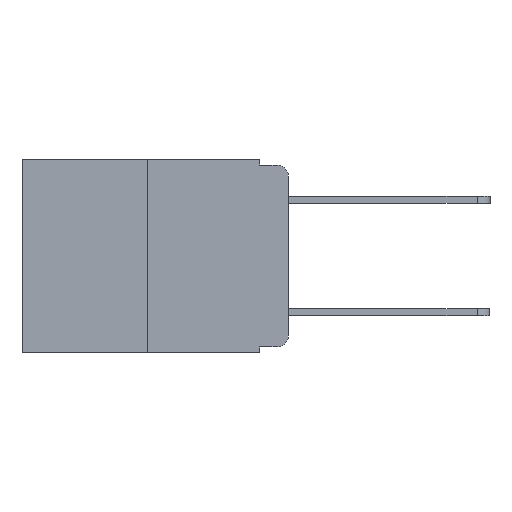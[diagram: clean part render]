
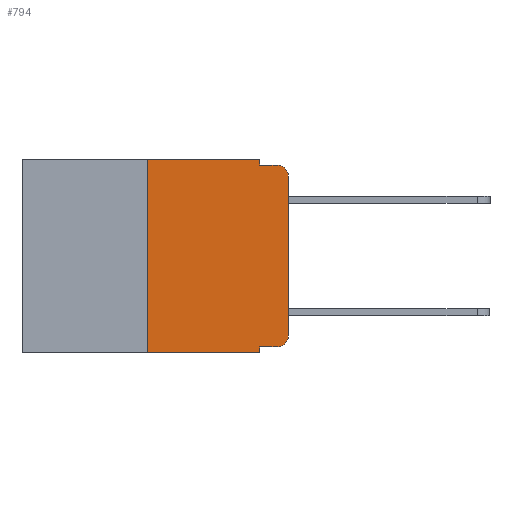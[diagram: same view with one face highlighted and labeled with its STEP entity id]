
A CAD part, left-side view. The second image highlights one B-rep face of the part: STEP entity #794.
In plain terms, the highlighted planar face has unit normal (-1, 0, 0).
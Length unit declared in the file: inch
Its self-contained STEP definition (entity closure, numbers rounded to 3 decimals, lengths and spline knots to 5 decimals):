
#40 = VERTEX_POINT ( 'NONE', #8375 ) ;
#88 = EDGE_CURVE ( 'NONE', #5300, #3965, #2626, .T. ) ;
#351 = ORIENTED_EDGE ( 'NONE', *, *, #1830, .T. ) ;
#376 = LINE ( 'NONE', #2778, #8539 ) ;
#382 = DIRECTION ( 'NONE',  ( 0., 0., -1. ) ) ;
#416 = DIRECTION ( 'NONE',  ( 1., 0., 0. ) ) ;
#794 = ADVANCED_FACE ( 'NONE', ( #3159 ), #2371, .F. ) ;
#861 = ORIENTED_EDGE ( 'NONE', *, *, #88, .F. ) ;
#867 = DIRECTION ( 'NONE',  ( 0., -1., 0. ) ) ;
#889 = ORIENTED_EDGE ( 'NONE', *, *, #10097, .T. ) ;
#949 = EDGE_CURVE ( 'NONE', #12232, #3965, #1345, .T. ) ;
#1345 = CIRCLE ( 'NONE', #6205, 0.02 ) ;
#1390 = LINE ( 'NONE', #2957, #11540 ) ;
#1554 = DIRECTION ( 'NONE',  ( 0., 0., 1. ) ) ;
#1636 = ORIENTED_EDGE ( 'NONE', *, *, #10668, .T. ) ;
#1830 = EDGE_CURVE ( 'NONE', #5233, #12232, #11865, .T. ) ;
#1864 = ORIENTED_EDGE ( 'NONE', *, *, #949, .T. ) ;
#2371 = PLANE ( 'NONE',  #11632 ) ;
#2626 = LINE ( 'NONE', #8330, #9819 ) ;
#2778 = CARTESIAN_POINT ( 'NONE',  ( 0., 0.051, 0. ) ) ;
#2957 = CARTESIAN_POINT ( 'NONE',  ( 0., 0.051, 0. ) ) ;
#3159 = FACE_OUTER_BOUND ( 'NONE', #12126, .T. ) ;
#3208 = EDGE_CURVE ( 'NONE', #40, #10435, #4902, .T. ) ;
#3879 = ORIENTED_EDGE ( 'NONE', *, *, #11744, .F. ) ;
#3965 = VERTEX_POINT ( 'NONE', #4578 ) ;
#3992 = DIRECTION ( 'NONE',  ( 0., -1., 0. ) ) ;
#4123 = DIRECTION ( 'NONE',  ( -1., 0., 0. ) ) ;
#4437 = VECTOR ( 'NONE', #867, 39.37008 ) ;
#4578 = CARTESIAN_POINT ( 'NONE',  ( 0., 0.02, -0.01 ) ) ;
#4671 = VECTOR ( 'NONE', #1554, 39.37008 ) ;
#4852 = VERTEX_POINT ( 'NONE', #12633 ) ;
#4874 = CARTESIAN_POINT ( 'NONE',  ( 0., 0., -0.03 ) ) ;
#4902 = LINE ( 'NONE', #9540, #6513 ) ;
#5088 = VECTOR ( 'NONE', #11750, 39.37008 ) ;
#5100 = CARTESIAN_POINT ( 'NONE',  ( 0., 0., 0. ) ) ;
#5233 = VERTEX_POINT ( 'NONE', #5254 ) ;
#5254 = CARTESIAN_POINT ( 'NONE',  ( 0., 0., -0.313 ) ) ;
#5300 = VERTEX_POINT ( 'NONE', #12439 ) ;
#5351 = ORIENTED_EDGE ( 'NONE', *, *, #11812, .F. ) ;
#5356 = CARTESIAN_POINT ( 'NONE',  ( 0., 0.051, -0.343 ) ) ;
#5508 = CARTESIAN_POINT ( 'NONE',  ( 0., 0.051, -0.333 ) ) ;
#6205 = AXIS2_PLACEMENT_3D ( 'NONE', #10348, #10448, #7154 ) ;
#6428 = CARTESIAN_POINT ( 'NONE',  ( 0., 0.473, 0. ) ) ;
#6513 = VECTOR ( 'NONE', #3992, 39.37008 ) ;
#7139 = CARTESIAN_POINT ( 'NONE',  ( 0., 0.473, 0. ) ) ;
#7154 = DIRECTION ( 'NONE',  ( 0., 0., -1. ) ) ;
#7412 = ORIENTED_EDGE ( 'NONE', *, *, #11241, .F. ) ;
#7468 = DIRECTION ( 'NONE',  ( 0., -1., 0. ) ) ;
#7708 = CIRCLE ( 'NONE', #11504, 0.02 ) ;
#8330 = CARTESIAN_POINT ( 'NONE',  ( 0., 0.051, -0.01 ) ) ;
#8375 = CARTESIAN_POINT ( 'NONE',  ( 0., 0.25, -0.343 ) ) ;
#8539 = VECTOR ( 'NONE', #8700, 39.37008 ) ;
#8700 = DIRECTION ( 'NONE',  ( 0., 0., -1. ) ) ;
#8958 = CARTESIAN_POINT ( 'NONE',  ( 0., 0.051, 0. ) ) ;
#9376 = LINE ( 'NONE', #5508, #4437 ) ;
#9540 = CARTESIAN_POINT ( 'NONE',  ( 0., 0.473, -0.343 ) ) ;
#9701 = CARTESIAN_POINT ( 'NONE',  ( 0., 0.02, -0.313 ) ) ;
#9735 = ORIENTED_EDGE ( 'NONE', *, *, #3208, .T. ) ;
#9737 = DIRECTION ( 'NONE',  ( 0., 0., -1. ) ) ;
#9819 = VECTOR ( 'NONE', #7468, 39.37008 ) ;
#9933 = LINE ( 'NONE', #10929, #11408 ) ;
#10073 = DIRECTION ( 'NONE',  ( 0., 0., 1. ) ) ;
#10097 = EDGE_CURVE ( 'NONE', #4852, #5233, #7708, .T. ) ;
#10136 = ORIENTED_EDGE ( 'NONE', *, *, #12410, .F. ) ;
#10348 = CARTESIAN_POINT ( 'NONE',  ( 0., 0.02, -0.03 ) ) ;
#10365 = VERTEX_POINT ( 'NONE', #8958 ) ;
#10435 = VERTEX_POINT ( 'NONE', #5356 ) ;
#10448 = DIRECTION ( 'NONE',  ( -1., 0., 0. ) ) ;
#10538 = VERTEX_POINT ( 'NONE', #10833 ) ;
#10570 = DIRECTION ( 'NONE',  ( 0., 0., -1. ) ) ;
#10668 = EDGE_CURVE ( 'NONE', #10538, #4852, #9376, .T. ) ;
#10833 = CARTESIAN_POINT ( 'NONE',  ( 0., 0.051, -0.333 ) ) ;
#10929 = CARTESIAN_POINT ( 'NONE',  ( 0., 0.25, 0. ) ) ;
#11241 = EDGE_CURVE ( 'NONE', #10538, #10435, #1390, .T. ) ;
#11408 = VECTOR ( 'NONE', #10073, 39.37008 ) ;
#11444 = VERTEX_POINT ( 'NONE', #12458 ) ;
#11504 = AXIS2_PLACEMENT_3D ( 'NONE', #9701, #4123, #10570 ) ;
#11540 = VECTOR ( 'NONE', #9737, 39.37008 ) ;
#11632 = AXIS2_PLACEMENT_3D ( 'NONE', #7139, #416, #382 ) ;
#11744 = EDGE_CURVE ( 'NONE', #11444, #10365, #11940, .T. ) ;
#11750 = DIRECTION ( 'NONE',  ( 0., -1., 0. ) ) ;
#11812 = EDGE_CURVE ( 'NONE', #40, #11444, #9933, .T. ) ;
#11865 = LINE ( 'NONE', #5100, #4671 ) ;
#11940 = LINE ( 'NONE', #6428, #5088 ) ;
#12126 = EDGE_LOOP ( 'NONE', ( #351, #1864, #861, #10136, #3879, #5351, #9735, #7412, #1636, #889 ) ) ;
#12232 = VERTEX_POINT ( 'NONE', #4874 ) ;
#12410 = EDGE_CURVE ( 'NONE', #10365, #5300, #376, .T. ) ;
#12439 = CARTESIAN_POINT ( 'NONE',  ( 0., 0.051, -0.01 ) ) ;
#12458 = CARTESIAN_POINT ( 'NONE',  ( 0., 0.25, 0. ) ) ;
#12633 = CARTESIAN_POINT ( 'NONE',  ( 0., 0.02, -0.333 ) ) ;
